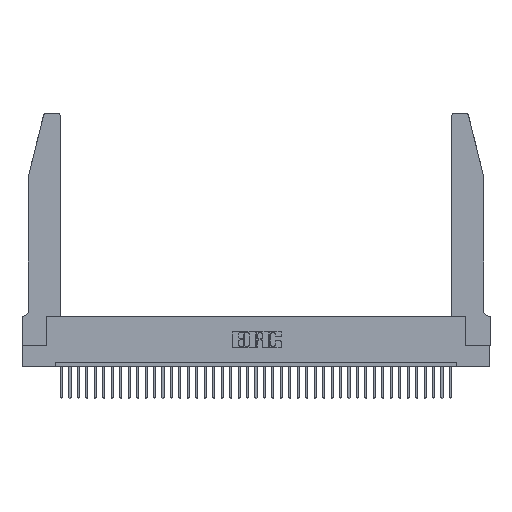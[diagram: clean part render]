
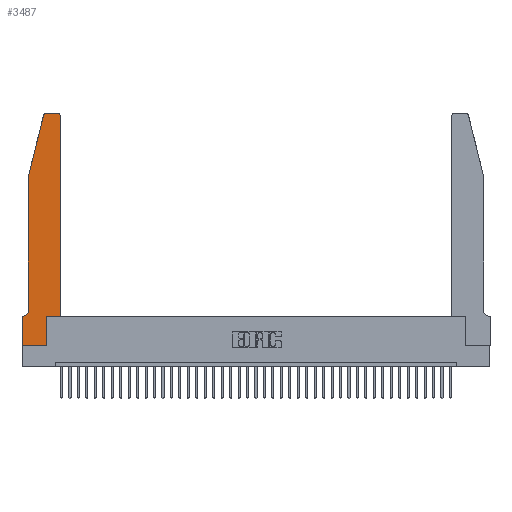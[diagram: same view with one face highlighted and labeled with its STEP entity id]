
A CAD part, top view. The second image highlights one B-rep face of the part: STEP entity #3487.
In plain terms, the highlighted planar face has unit normal (0, 0, 1).
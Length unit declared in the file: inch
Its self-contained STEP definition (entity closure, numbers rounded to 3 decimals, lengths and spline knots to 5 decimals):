
#274 = ORIENTED_EDGE ( 'NONE', *, *, #13070, .T. ) ;
#336 = VERTEX_POINT ( 'NONE', #24759 ) ;
#436 = LINE ( 'NONE', #2207, #39031 ) ;
#1274 = DIRECTION ( 'NONE',  ( 1., 0., 0. ) ) ;
#1448 = DIRECTION ( 'NONE',  ( -1., 0., 0. ) ) ;
#2175 = DIRECTION ( 'NONE',  ( 1., 0., 0. ) ) ;
#2186 = CIRCLE ( 'NONE', #32936, 0.07 ) ;
#2207 = CARTESIAN_POINT ( 'NONE',  ( 0.2865, 0.35, 0.37 ) ) ;
#2430 = CARTESIAN_POINT ( 'NONE',  ( 0.0755, 2., 0.37 ) ) ;
#2636 = VECTOR ( 'NONE', #2654, 39.37008 ) ;
#2654 = DIRECTION ( 'NONE',  ( -0.239, -0.971, 0. ) ) ;
#2865 = ORIENTED_EDGE ( 'NONE', *, *, #20566, .T. ) ;
#2898 = VERTEX_POINT ( 'NONE', #22732 ) ;
#3487 = ADVANCED_FACE ( 'NONE', ( #34014 ), #38513, .T. ) ;
#3714 = DIRECTION ( 'NONE',  ( 0., 0., 1. ) ) ;
#3751 = EDGE_CURVE ( 'NONE', #21793, #20444, #5386, .T. ) ;
#4109 = VECTOR ( 'NONE', #1274, 39.37008 ) ;
#4511 = DIRECTION ( 'NONE',  ( 0., 0., -1. ) ) ;
#4532 = EDGE_CURVE ( 'NONE', #26503, #38818, #31684, .T. ) ;
#4785 = ORIENTED_EDGE ( 'NONE', *, *, #18515, .T. ) ;
#4899 = ORIENTED_EDGE ( 'NONE', *, *, #3751, .T. ) ;
#5386 = LINE ( 'NONE', #26103, #8246 ) ;
#6427 = CARTESIAN_POINT ( 'NONE',  ( 0.4505, 0.35, 0.37 ) ) ;
#6994 = ORIENTED_EDGE ( 'NONE', *, *, #23574, .T. ) ;
#7077 = CARTESIAN_POINT ( 'NONE',  ( 0.0755, 2., 0.37 ) ) ;
#7706 = VERTEX_POINT ( 'NONE', #27765 ) ;
#8029 = DIRECTION ( 'NONE',  ( 0., 0., 1. ) ) ;
#8246 = VECTOR ( 'NONE', #25586, 39.37008 ) ;
#8902 = VECTOR ( 'NONE', #34810, 39.37008 ) ;
#9635 = EDGE_CURVE ( 'NONE', #26194, #7706, #436, .T. ) ;
#10326 = AXIS2_PLACEMENT_3D ( 'NONE', #11355, #8029, #2175 ) ;
#10525 = CARTESIAN_POINT ( 'NONE',  ( 0.2865, 0., 0.37 ) ) ;
#11233 = CIRCLE ( 'NONE', #10326, 0.03 ) ;
#11355 = CARTESIAN_POINT ( 'NONE',  ( 0.284, 2.72, 0.37 ) ) ;
#11459 = DIRECTION ( 'NONE',  ( 1., 0., 0. ) ) ;
#11779 = VECTOR ( 'NONE', #16044, 39.37008 ) ;
#11964 = LINE ( 'NONE', #28882, #38669 ) ;
#12352 = EDGE_CURVE ( 'NONE', #2898, #26020, #14710, .T. ) ;
#12442 = ORIENTED_EDGE ( 'NONE', *, *, #26332, .T. ) ;
#13070 = EDGE_CURVE ( 'NONE', #336, #21793, #21253, .T. ) ;
#13207 = CARTESIAN_POINT ( 'NONE',  ( 0.2605, 2.75, 0.37 ) ) ;
#13320 = EDGE_CURVE ( 'NONE', #26020, #20468, #31271, .T. ) ;
#13916 = DIRECTION ( 'NONE',  ( 0., 1., 0. ) ) ;
#14710 = LINE ( 'NONE', #6427, #33312 ) ;
#14889 = DIRECTION ( 'NONE',  ( 0., 0., 1. ) ) ;
#15710 = DIRECTION ( 'NONE',  ( 0., 1., 0. ) ) ;
#16044 = DIRECTION ( 'NONE',  ( -1., 0., 0. ) ) ;
#16472 = CARTESIAN_POINT ( 'NONE',  ( 0.0055, 0.42, 0.37 ) ) ;
#17946 = DIRECTION ( 'NONE',  ( 1., 0., 0. ) ) ;
#18151 = ORIENTED_EDGE ( 'NONE', *, *, #13320, .T. ) ;
#18490 = ORIENTED_EDGE ( 'NONE', *, *, #25450, .T. ) ;
#18515 = EDGE_CURVE ( 'NONE', #20468, #37890, #34165, .T. ) ;
#19702 = CARTESIAN_POINT ( 'NONE',  ( 0., 0.35, 0.37 ) ) ;
#20444 = VERTEX_POINT ( 'NONE', #27601 ) ;
#20468 = VERTEX_POINT ( 'NONE', #27859 ) ;
#20566 = EDGE_CURVE ( 'NONE', #38818, #27286, #33027, .T. ) ;
#20927 = AXIS2_PLACEMENT_3D ( 'NONE', #26974, #14889, #17946 ) ;
#21253 = LINE ( 'NONE', #28025, #11779 ) ;
#21531 = AXIS2_PLACEMENT_3D ( 'NONE', #21887, #3714, #28854 ) ;
#21793 = VERTEX_POINT ( 'NONE', #19702 ) ;
#21887 = CARTESIAN_POINT ( 'NONE',  ( 0.4205, 2.72, 0.37 ) ) ;
#21989 = VECTOR ( 'NONE', #38942, 39.37008 ) ;
#22732 = CARTESIAN_POINT ( 'NONE',  ( 0.4505, 0.35, 0.37 ) ) ;
#23093 = ORIENTED_EDGE ( 'NONE', *, *, #4532, .T. ) ;
#23574 = EDGE_CURVE ( 'NONE', #20444, #26194, #11964, .T. ) ;
#24619 = CARTESIAN_POINT ( 'NONE',  ( 0.4505, 2.72, 0.37 ) ) ;
#24731 = EDGE_LOOP ( 'NONE', ( #4785, #25476, #23093, #2865, #12442, #274, #4899, #6994, #28387, #18490, #25486, #18151 ) ) ;
#24759 = CARTESIAN_POINT ( 'NONE',  ( 0.0055, 0.35, 0.37 ) ) ;
#25450 = EDGE_CURVE ( 'NONE', #7706, #2898, #28860, .T. ) ;
#25476 = ORIENTED_EDGE ( 'NONE', *, *, #28796, .T. ) ;
#25486 = ORIENTED_EDGE ( 'NONE', *, *, #12352, .T. ) ;
#25586 = DIRECTION ( 'NONE',  ( 0., -1., 0. ) ) ;
#26020 = VERTEX_POINT ( 'NONE', #24619 ) ;
#26103 = CARTESIAN_POINT ( 'NONE',  ( 0., 0., 0.37 ) ) ;
#26194 = VERTEX_POINT ( 'NONE', #10525 ) ;
#26332 = EDGE_CURVE ( 'NONE', #27286, #336, #2186, .T. ) ;
#26503 = VERTEX_POINT ( 'NONE', #32448 ) ;
#26562 = CARTESIAN_POINT ( 'NONE',  ( 0.284, 2.75, 0.37 ) ) ;
#26974 = CARTESIAN_POINT ( 'NONE',  ( 0., 0.35, 0.37 ) ) ;
#27286 = VERTEX_POINT ( 'NONE', #33746 ) ;
#27601 = CARTESIAN_POINT ( 'NONE',  ( 0., 0., 0.37 ) ) ;
#27765 = CARTESIAN_POINT ( 'NONE',  ( 0.2865, 0.35, 0.37 ) ) ;
#27859 = CARTESIAN_POINT ( 'NONE',  ( 0.4205, 2.75, 0.37 ) ) ;
#28025 = CARTESIAN_POINT ( 'NONE',  ( 0.0755, 0.35, 0.37 ) ) ;
#28274 = CARTESIAN_POINT ( 'NONE',  ( 0.4505, 0.35, 0.37 ) ) ;
#28387 = ORIENTED_EDGE ( 'NONE', *, *, #9635, .T. ) ;
#28796 = EDGE_CURVE ( 'NONE', #37890, #26503, #11233, .T. ) ;
#28854 = DIRECTION ( 'NONE',  ( 1., 0., 0. ) ) ;
#28860 = LINE ( 'NONE', #28274, #4109 ) ;
#28882 = CARTESIAN_POINT ( 'NONE',  ( 0., 0., 0.37 ) ) ;
#31271 = CIRCLE ( 'NONE', #21531, 0.03 ) ;
#31684 = LINE ( 'NONE', #35446, #2636 ) ;
#32448 = CARTESIAN_POINT ( 'NONE',  ( 0.25487, 2.72718, 0.37 ) ) ;
#32936 = AXIS2_PLACEMENT_3D ( 'NONE', #16472, #4511, #1448 ) ;
#33027 = LINE ( 'NONE', #2430, #21989 ) ;
#33312 = VECTOR ( 'NONE', #15710, 39.37008 ) ;
#33746 = CARTESIAN_POINT ( 'NONE',  ( 0.0755, 0.42, 0.37 ) ) ;
#34014 = FACE_OUTER_BOUND ( 'NONE', #24731, .T. ) ;
#34165 = LINE ( 'NONE', #13207, #8902 ) ;
#34810 = DIRECTION ( 'NONE',  ( -1., 0., 0. ) ) ;
#35446 = CARTESIAN_POINT ( 'NONE',  ( 0.0755, 2., 0.37 ) ) ;
#37890 = VERTEX_POINT ( 'NONE', #26562 ) ;
#38513 = PLANE ( 'NONE',  #20927 ) ;
#38669 = VECTOR ( 'NONE', #11459, 39.37008 ) ;
#38818 = VERTEX_POINT ( 'NONE', #7077 ) ;
#38942 = DIRECTION ( 'NONE',  ( 0., -1., 0. ) ) ;
#39031 = VECTOR ( 'NONE', #13916, 39.37008 ) ;
